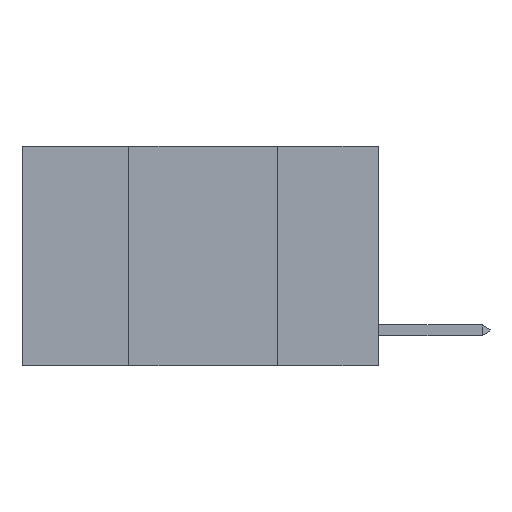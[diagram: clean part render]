
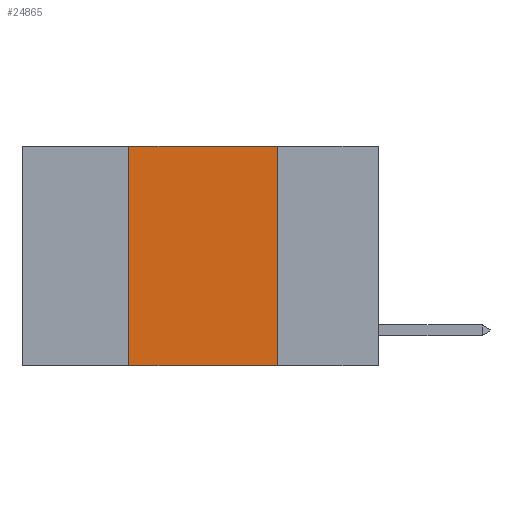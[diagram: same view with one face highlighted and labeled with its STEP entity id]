
A CAD part, left-side view. The second image highlights one B-rep face of the part: STEP entity #24865.
In plain terms, the highlighted planar face has unit normal (-1, 0, 0).
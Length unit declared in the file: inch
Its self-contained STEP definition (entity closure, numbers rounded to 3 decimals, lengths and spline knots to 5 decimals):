
#970 = VERTEX_POINT ( 'NONE', #9807 ) ;
#1132 = CARTESIAN_POINT ( 'NONE',  ( 0., 0.6, -0.37 ) ) ;
#1848 = CARTESIAN_POINT ( 'NONE',  ( 0., 0.42, -0.37 ) ) ;
#1991 = VERTEX_POINT ( 'NONE', #12340 ) ;
#2112 = ORIENTED_EDGE ( 'NONE', *, *, #8425, .T. ) ;
#4671 = LINE ( 'NONE', #1132, #11711 ) ;
#5328 = DIRECTION ( 'NONE',  ( 0., 0., 1. ) ) ;
#5488 = LINE ( 'NONE', #14395, #24634 ) ;
#6287 = DIRECTION ( 'NONE',  ( 0., 0., -1. ) ) ;
#7018 = AXIS2_PLACEMENT_3D ( 'NONE', #15354, #22281, #6287 ) ;
#7457 = VECTOR ( 'NONE', #23284, 39.37008 ) ;
#8367 = VERTEX_POINT ( 'NONE', #19100 ) ;
#8425 = EDGE_CURVE ( 'NONE', #20641, #8367, #4671, .T. ) ;
#8784 = FACE_OUTER_BOUND ( 'NONE', #22083, .T. ) ;
#8864 = LINE ( 'NONE', #14276, #7457 ) ;
#9807 = CARTESIAN_POINT ( 'NONE',  ( 0., 0.17, 0. ) ) ;
#11377 = LINE ( 'NONE', #15348, #28771 ) ;
#11711 = VECTOR ( 'NONE', #14919, 39.37008 ) ;
#12340 = CARTESIAN_POINT ( 'NONE',  ( 0., 0.42, 0. ) ) ;
#13669 = ORIENTED_EDGE ( 'NONE', *, *, #28385, .F. ) ;
#14276 = CARTESIAN_POINT ( 'NONE',  ( 0., 0.17, 0. ) ) ;
#14395 = CARTESIAN_POINT ( 'NONE',  ( 0., 0.42, 0. ) ) ;
#14413 = ORIENTED_EDGE ( 'NONE', *, *, #15256, .F. ) ;
#14919 = DIRECTION ( 'NONE',  ( 0., -1., 0. ) ) ;
#15256 = EDGE_CURVE ( 'NONE', #1991, #970, #11377, .T. ) ;
#15348 = CARTESIAN_POINT ( 'NONE',  ( 0., 0.6, 0. ) ) ;
#15354 = CARTESIAN_POINT ( 'NONE',  ( 0., 0.6, 0. ) ) ;
#18038 = DIRECTION ( 'NONE',  ( 0., -1., 0. ) ) ;
#19100 = CARTESIAN_POINT ( 'NONE',  ( 0., 0.17, -0.37 ) ) ;
#19338 = PLANE ( 'NONE',  #7018 ) ;
#20641 = VERTEX_POINT ( 'NONE', #1848 ) ;
#21033 = ORIENTED_EDGE ( 'NONE', *, *, #21397, .F. ) ;
#21397 = EDGE_CURVE ( 'NONE', #20641, #1991, #5488, .T. ) ;
#22083 = EDGE_LOOP ( 'NONE', ( #13669, #14413, #21033, #2112 ) ) ;
#22281 = DIRECTION ( 'NONE',  ( 1., 0., 0. ) ) ;
#23284 = DIRECTION ( 'NONE',  ( 0., 0., -1. ) ) ;
#24634 = VECTOR ( 'NONE', #5328, 39.37008 ) ;
#24865 = ADVANCED_FACE ( 'NONE', ( #8784 ), #19338, .F. ) ;
#28385 = EDGE_CURVE ( 'NONE', #970, #8367, #8864, .T. ) ;
#28771 = VECTOR ( 'NONE', #18038, 39.37008 ) ;
